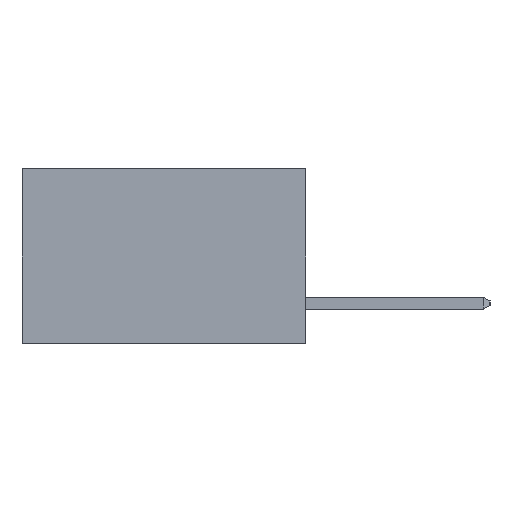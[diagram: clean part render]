
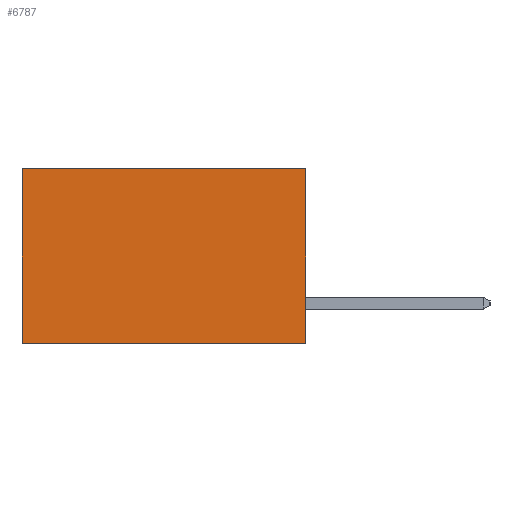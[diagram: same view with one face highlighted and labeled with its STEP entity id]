
A CAD part, left-side view. The second image highlights one B-rep face of the part: STEP entity #6787.
In plain terms, the highlighted planar face has unit normal (-1, 0, 0).
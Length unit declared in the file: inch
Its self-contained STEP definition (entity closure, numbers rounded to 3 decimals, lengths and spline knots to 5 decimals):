
#189 = LINE ( 'NONE', #8769, #2585 ) ;
#337 = VERTEX_POINT ( 'NONE', #5990 ) ;
#681 = VERTEX_POINT ( 'NONE', #9666 ) ;
#1244 = VECTOR ( 'NONE', #6325, 39.37008 ) ;
#1246 = CARTESIAN_POINT ( 'NONE',  ( 0.2615, 0., -0.37 ) ) ;
#1603 = ORIENTED_EDGE ( 'NONE', *, *, #3554, .T. ) ;
#2585 = VECTOR ( 'NONE', #8730, 39.37008 ) ;
#2786 = FACE_OUTER_BOUND ( 'NONE', #5224, .T. ) ;
#2851 = DIRECTION ( 'NONE',  ( 0., 0., -1. ) ) ;
#3085 = VERTEX_POINT ( 'NONE', #4553 ) ;
#3501 = EDGE_CURVE ( 'NONE', #337, #8658, #189, .T. ) ;
#3554 = EDGE_CURVE ( 'NONE', #8658, #681, #11291, .T. ) ;
#4037 = VECTOR ( 'NONE', #2851, 39.37008 ) ;
#4381 = CARTESIAN_POINT ( 'NONE',  ( 0.2615, 0.6, 0. ) ) ;
#4553 = CARTESIAN_POINT ( 'NONE',  ( 0.2615, 0., -0.37 ) ) ;
#5216 = DIRECTION ( 'NONE',  ( 0., 0., -1. ) ) ;
#5224 = EDGE_LOOP ( 'NONE', ( #1603, #6626, #11237, #6915 ) ) ;
#5302 = EDGE_CURVE ( 'NONE', #337, #3085, #6527, .T. ) ;
#5479 = CARTESIAN_POINT ( 'NONE',  ( 0.2615, 0.6, -0.37 ) ) ;
#5990 = CARTESIAN_POINT ( 'NONE',  ( 0.2615, 0., 0. ) ) ;
#6149 = CARTESIAN_POINT ( 'NONE',  ( 0.2615, 0., -0.37 ) ) ;
#6325 = DIRECTION ( 'NONE',  ( 0., 1., 0. ) ) ;
#6527 = LINE ( 'NONE', #1246, #4037 ) ;
#6626 = ORIENTED_EDGE ( 'NONE', *, *, #8568, .F. ) ;
#6768 = CARTESIAN_POINT ( 'NONE',  ( 0.2615, 0., -0.37 ) ) ;
#6787 = ADVANCED_FACE ( 'NONE', ( #2786 ), #8914, .F. ) ;
#6915 = ORIENTED_EDGE ( 'NONE', *, *, #3501, .T. ) ;
#7131 = DIRECTION ( 'NONE',  ( 0., 0., -1. ) ) ;
#7136 = DIRECTION ( 'NONE',  ( 1., 0., 0. ) ) ;
#8568 = EDGE_CURVE ( 'NONE', #3085, #681, #10678, .T. ) ;
#8658 = VERTEX_POINT ( 'NONE', #4381 ) ;
#8730 = DIRECTION ( 'NONE',  ( 0., 1., 0. ) ) ;
#8769 = CARTESIAN_POINT ( 'NONE',  ( 0.2615, 0., 0. ) ) ;
#8914 = PLANE ( 'NONE',  #9857 ) ;
#9317 = VECTOR ( 'NONE', #5216, 39.37008 ) ;
#9666 = CARTESIAN_POINT ( 'NONE',  ( 0.2615, 0.6, -0.37 ) ) ;
#9857 = AXIS2_PLACEMENT_3D ( 'NONE', #6768, #7136, #7131 ) ;
#10678 = LINE ( 'NONE', #6149, #1244 ) ;
#11237 = ORIENTED_EDGE ( 'NONE', *, *, #5302, .F. ) ;
#11291 = LINE ( 'NONE', #5479, #9317 ) ;
